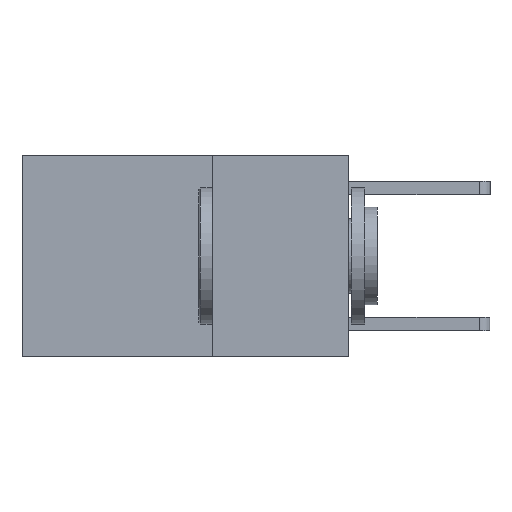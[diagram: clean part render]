
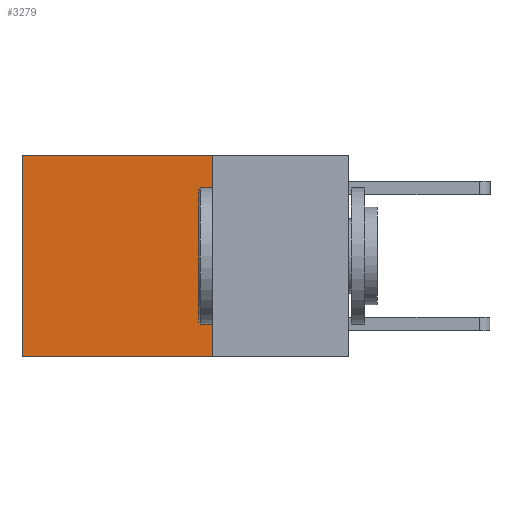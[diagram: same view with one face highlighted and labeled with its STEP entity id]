
A CAD part, left-side view. The second image highlights one B-rep face of the part: STEP entity #3279.
In plain terms, the highlighted planar face has unit normal (-1, 0, 0).
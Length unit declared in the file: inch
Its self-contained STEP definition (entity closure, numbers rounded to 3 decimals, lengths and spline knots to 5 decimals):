
#9 = DIRECTION ( 'NONE',  ( 1., 0., 0. ) ) ;
#38 = VECTOR ( 'NONE', #8138, 39.37008 ) ;
#611 = EDGE_CURVE ( 'NONE', #2833, #3160, #2989, .T. ) ;
#774 = EDGE_CURVE ( 'NONE', #2833, #8290, #3080, .T. ) ;
#780 = CARTESIAN_POINT ( 'NONE',  ( 0.2625, 0.6, 0. ) ) ;
#865 = CARTESIAN_POINT ( 'NONE',  ( 0.2625, 0.25, 0. ) ) ;
#1629 = CARTESIAN_POINT ( 'NONE',  ( 0.2625, 0.25, 0. ) ) ;
#1804 = CARTESIAN_POINT ( 'NONE',  ( 0.2625, 0.25, 0. ) ) ;
#2207 = DIRECTION ( 'NONE',  ( 0., 0., -1. ) ) ;
#2538 = ORIENTED_EDGE ( 'NONE', *, *, #7001, .T. ) ;
#2609 = LINE ( 'NONE', #6814, #2765 ) ;
#2765 = VECTOR ( 'NONE', #3208, 39.37008 ) ;
#2833 = VERTEX_POINT ( 'NONE', #1804 ) ;
#2887 = VECTOR ( 'NONE', #2950, 39.37008 ) ;
#2950 = DIRECTION ( 'NONE',  ( 0., 1., 0. ) ) ;
#2989 = LINE ( 'NONE', #865, #2887 ) ;
#3080 = LINE ( 'NONE', #1629, #38 ) ;
#3160 = VERTEX_POINT ( 'NONE', #9068 ) ;
#3195 = ORIENTED_EDGE ( 'NONE', *, *, #611, .T. ) ;
#3208 = DIRECTION ( 'NONE',  ( 0., 1., 0. ) ) ;
#3279 = ADVANCED_FACE ( 'NONE', ( #5659 ), #5610, .F. ) ;
#3487 = ORIENTED_EDGE ( 'NONE', *, *, #4926, .F. ) ;
#3999 = CARTESIAN_POINT ( 'NONE',  ( 0.2625, 0.25, -0.37 ) ) ;
#4926 = EDGE_CURVE ( 'NONE', #8290, #5894, #2609, .T. ) ;
#5610 = PLANE ( 'NONE',  #8202 ) ;
#5659 = FACE_OUTER_BOUND ( 'NONE', #6028, .T. ) ;
#5696 = CARTESIAN_POINT ( 'NONE',  ( 0.2625, 0.6, -0.37 ) ) ;
#5771 = ORIENTED_EDGE ( 'NONE', *, *, #774, .F. ) ;
#5894 = VERTEX_POINT ( 'NONE', #5696 ) ;
#6028 = EDGE_LOOP ( 'NONE', ( #2538, #3487, #5771, #3195 ) ) ;
#6312 = CARTESIAN_POINT ( 'NONE',  ( 0.2625, 0.25, 0. ) ) ;
#6814 = CARTESIAN_POINT ( 'NONE',  ( 0.2625, 0.25, -0.37 ) ) ;
#7001 = EDGE_CURVE ( 'NONE', #3160, #5894, #8617, .T. ) ;
#8084 = VECTOR ( 'NONE', #2207, 39.37008 ) ;
#8138 = DIRECTION ( 'NONE',  ( 0., 0., -1. ) ) ;
#8202 = AXIS2_PLACEMENT_3D ( 'NONE', #6312, #9, #9202 ) ;
#8290 = VERTEX_POINT ( 'NONE', #3999 ) ;
#8617 = LINE ( 'NONE', #780, #8084 ) ;
#9068 = CARTESIAN_POINT ( 'NONE',  ( 0.2625, 0.6, 0. ) ) ;
#9202 = DIRECTION ( 'NONE',  ( 0., 0., -1. ) ) ;
